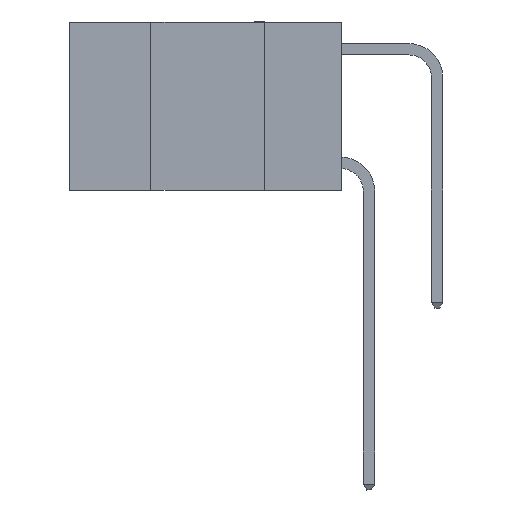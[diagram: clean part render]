
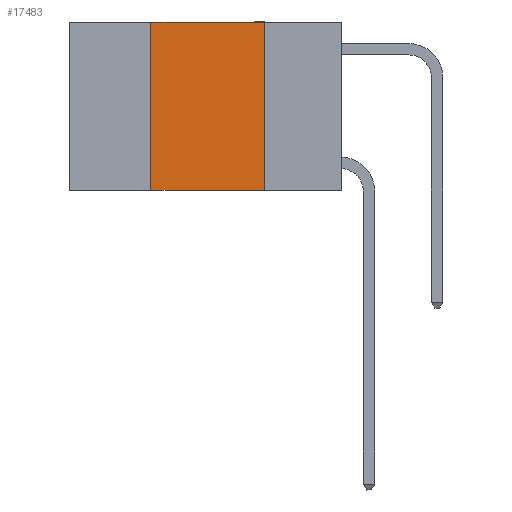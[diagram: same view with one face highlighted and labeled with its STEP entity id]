
A CAD part, left-side view. The second image highlights one B-rep face of the part: STEP entity #17483.
In plain terms, the highlighted planar face has unit normal (-1, 0, 0).
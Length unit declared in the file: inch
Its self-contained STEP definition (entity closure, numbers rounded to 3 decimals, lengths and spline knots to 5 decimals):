
#473 = DIRECTION ( 'NONE',  ( 0., -1., 0. ) ) ;
#1495 = EDGE_CURVE ( 'NONE', #15402, #21710, #15825, .T. ) ;
#2135 = DIRECTION ( 'NONE',  ( 0., 0., 1. ) ) ;
#2558 = ORIENTED_EDGE ( 'NONE', *, *, #20944, .F. ) ;
#3165 = CARTESIAN_POINT ( 'NONE',  ( 0., 0.17, 0. ) ) ;
#3391 = ORIENTED_EDGE ( 'NONE', *, *, #1495, .F. ) ;
#7336 = VERTEX_POINT ( 'NONE', #13119 ) ;
#7565 = CARTESIAN_POINT ( 'NONE',  ( 0., 0.6, -0.37 ) ) ;
#7837 = FACE_OUTER_BOUND ( 'NONE', #17716, .T. ) ;
#10170 = CARTESIAN_POINT ( 'NONE',  ( 0., 0.42, -0.37 ) ) ;
#10390 = VECTOR ( 'NONE', #473, 39.37008 ) ;
#11340 = DIRECTION ( 'NONE',  ( 0., -1., 0. ) ) ;
#11633 = AXIS2_PLACEMENT_3D ( 'NONE', #16825, #22327, #20230 ) ;
#11678 = VECTOR ( 'NONE', #11340, 39.37008 ) ;
#13119 = CARTESIAN_POINT ( 'NONE',  ( 0., 0.42, 0. ) ) ;
#13307 = PLANE ( 'NONE',  #11633 ) ;
#14165 = EDGE_CURVE ( 'NONE', #7336, #15402, #23007, .T. ) ;
#14813 = ORIENTED_EDGE ( 'NONE', *, *, #19123, .T. ) ;
#15167 = CARTESIAN_POINT ( 'NONE',  ( 0., 0.42, 0. ) ) ;
#15402 = VERTEX_POINT ( 'NONE', #21252 ) ;
#15825 = LINE ( 'NONE', #3165, #20114 ) ;
#16825 = CARTESIAN_POINT ( 'NONE',  ( 0., 0.6, 0. ) ) ;
#17101 = LINE ( 'NONE', #15167, #22197 ) ;
#17282 = CARTESIAN_POINT ( 'NONE',  ( 0., 0.6, 0. ) ) ;
#17483 = ADVANCED_FACE ( 'NONE', ( #7837 ), #13307, .F. ) ;
#17716 = EDGE_LOOP ( 'NONE', ( #3391, #21241, #2558, #14813 ) ) ;
#17836 = CARTESIAN_POINT ( 'NONE',  ( 0., 0.17, -0.37 ) ) ;
#19123 = EDGE_CURVE ( 'NONE', #22998, #21710, #22537, .T. ) ;
#20114 = VECTOR ( 'NONE', #23364, 39.37008 ) ;
#20230 = DIRECTION ( 'NONE',  ( 0., 0., -1. ) ) ;
#20944 = EDGE_CURVE ( 'NONE', #22998, #7336, #17101, .T. ) ;
#21241 = ORIENTED_EDGE ( 'NONE', *, *, #14165, .F. ) ;
#21252 = CARTESIAN_POINT ( 'NONE',  ( 0., 0.17, 0. ) ) ;
#21710 = VERTEX_POINT ( 'NONE', #17836 ) ;
#22197 = VECTOR ( 'NONE', #2135, 39.37008 ) ;
#22327 = DIRECTION ( 'NONE',  ( 1., 0., 0. ) ) ;
#22537 = LINE ( 'NONE', #7565, #11678 ) ;
#22998 = VERTEX_POINT ( 'NONE', #10170 ) ;
#23007 = LINE ( 'NONE', #17282, #10390 ) ;
#23364 = DIRECTION ( 'NONE',  ( 0., 0., -1. ) ) ;
